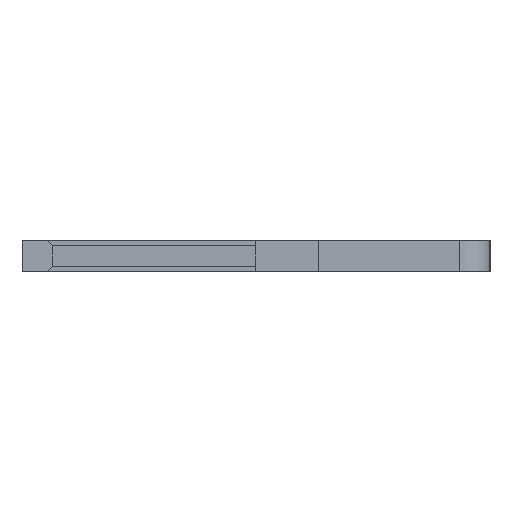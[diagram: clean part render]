
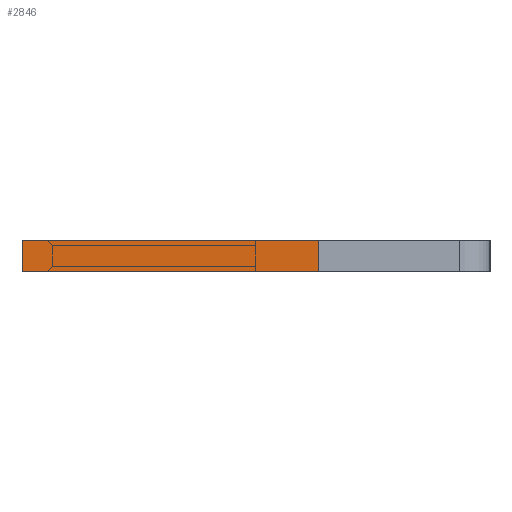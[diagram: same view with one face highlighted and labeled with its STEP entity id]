
A CAD part, left-side view. The second image highlights one B-rep face of the part: STEP entity #2846.
In plain terms, the highlighted face is planar.
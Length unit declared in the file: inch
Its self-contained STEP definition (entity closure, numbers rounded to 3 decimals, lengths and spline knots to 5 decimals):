
#3 = CARTESIAN_POINT ( 'NONE',  ( 0.01, 0.15, -0.04 ) ) ;
#194 = VERTEX_POINT ( 'NONE', #2501 ) ;
#229 = CARTESIAN_POINT ( 'NONE',  ( 0.01, 0.15, -0.04 ) ) ;
#304 = EDGE_LOOP ( 'NONE', ( #491, #3311, #905, #2315 ) ) ;
#380 = PLANE ( 'NONE',  #1831 ) ;
#491 = ORIENTED_EDGE ( 'NONE', *, *, #3403, .T. ) ;
#622 = CARTESIAN_POINT ( 'NONE',  ( 0.01, 0.15, -0.04 ) ) ;
#726 = CARTESIAN_POINT ( 'NONE',  ( 0.01, -0.04, -0.04 ) ) ;
#772 = VECTOR ( 'NONE', #2748, 39.37008 ) ;
#845 = DIRECTION ( 'NONE',  ( 0., 1., 0. ) ) ;
#905 = ORIENTED_EDGE ( 'NONE', *, *, #2093, .F. ) ;
#929 = CARTESIAN_POINT ( 'NONE',  ( 0.01, 0.15, -0.04 ) ) ;
#961 = VERTEX_POINT ( 'NONE', #229 ) ;
#1147 = VECTOR ( 'NONE', #845, 39.37008 ) ;
#1233 = CARTESIAN_POINT ( 'NONE',  ( -0.01, -0.04, -0.04 ) ) ;
#1500 = DIRECTION ( 'NONE',  ( 0., 0., 1. ) ) ;
#1831 = AXIS2_PLACEMENT_3D ( 'NONE', #929, #1500, #2395 ) ;
#1989 = VECTOR ( 'NONE', #3611, 39.37008 ) ;
#2093 = EDGE_CURVE ( 'NONE', #2949, #961, #3461, .T. ) ;
#2176 = CARTESIAN_POINT ( 'NONE',  ( -0.01, 0.15, -0.04 ) ) ;
#2315 = ORIENTED_EDGE ( 'NONE', *, *, #2947, .T. ) ;
#2395 = DIRECTION ( 'NONE',  ( 1., 0., 0. ) ) ;
#2414 = CARTESIAN_POINT ( 'NONE',  ( 0.01, -0.04, -0.04 ) ) ;
#2501 = CARTESIAN_POINT ( 'NONE',  ( -0.01, 0.15, -0.04 ) ) ;
#2509 = LINE ( 'NONE', #2176, #1989 ) ;
#2714 = VERTEX_POINT ( 'NONE', #1233 ) ;
#2728 = LINE ( 'NONE', #622, #3418 ) ;
#2748 = DIRECTION ( 'NONE',  ( -1., 0., 0. ) ) ;
#2804 = LINE ( 'NONE', #726, #772 ) ;
#2846 = ADVANCED_FACE ( 'NONE', ( #3324 ), #380, .F. ) ;
#2875 = EDGE_CURVE ( 'NONE', #961, #194, #2728, .T. ) ;
#2947 = EDGE_CURVE ( 'NONE', #2949, #2714, #2804, .T. ) ;
#2949 = VERTEX_POINT ( 'NONE', #2414 ) ;
#3311 = ORIENTED_EDGE ( 'NONE', *, *, #2875, .F. ) ;
#3324 = FACE_OUTER_BOUND ( 'NONE', #304, .T. ) ;
#3403 = EDGE_CURVE ( 'NONE', #2714, #194, #2509, .T. ) ;
#3418 = VECTOR ( 'NONE', #3522, 39.37008 ) ;
#3461 = LINE ( 'NONE', #3, #1147 ) ;
#3522 = DIRECTION ( 'NONE',  ( -1., 0., 0. ) ) ;
#3611 = DIRECTION ( 'NONE',  ( 0., 1., 0. ) ) ;
